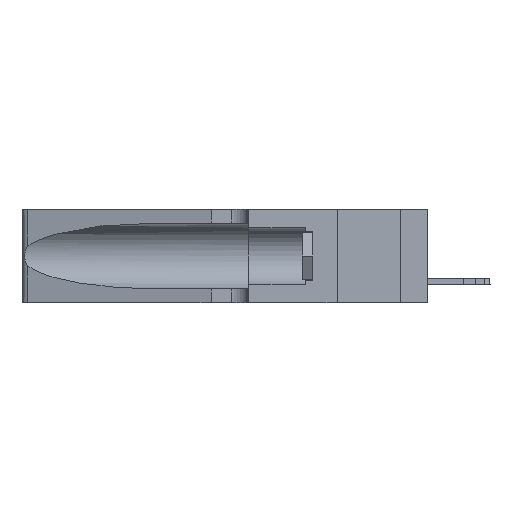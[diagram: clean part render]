
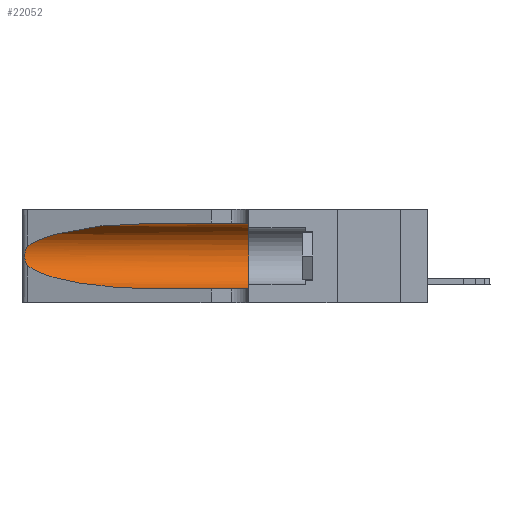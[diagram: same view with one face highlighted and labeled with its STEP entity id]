
A CAD part, left-side view. The second image highlights one B-rep face of the part: STEP entity #22052.
In plain terms, the highlighted cylindrical face has radius 3.308 mm (diameter 6.617 mm), a partial arc.
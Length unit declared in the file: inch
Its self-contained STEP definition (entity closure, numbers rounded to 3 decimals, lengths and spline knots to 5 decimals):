
#426 = CARTESIAN_POINT ( 'NONE',  ( 0.1305, 1.61858, 0.185 ) ) ;
#627 = CARTESIAN_POINT ( 'NONE',  ( 0.1305, 1.61858, 0.05475 ) ) ;
#1019 = EDGE_CURVE ( 'NONE', #13093, #15807, #2407, .T. ) ;
#1480 = CARTESIAN_POINT ( 'NONE',  ( 0.1305, 0.35, 0.31525 ) ) ;
#1628 = CARTESIAN_POINT ( 'NONE',  ( 0.26075, 1.23896, 0.19203 ) ) ;
#2133 = EDGE_CURVE ( 'NONE', #15807, #19721, #5333, .T. ) ;
#2407 =( BOUNDED_CURVE ( )  B_SPLINE_CURVE ( 3, ( #13486, #13326, #16938, #17196 ),
 .UNSPECIFIED., .F., .T. ) 
 B_SPLINE_CURVE_WITH_KNOTS ( ( 4, 4 ),
 ( 3.44316, 4.71239 ),
 .UNSPECIFIED. ) 
 CURVE ( )  GEOMETRIC_REPRESENTATION_ITEM ( )  RATIONAL_B_SPLINE_CURVE ( ( 1., 0.87, 0.87, 1. ) ) 
 REPRESENTATION_ITEM ( '' )  );
#2985 = ORIENTED_EDGE ( 'NONE', *, *, #22074, .T. ) ;
#3859 = CARTESIAN_POINT ( 'NONE',  ( 0.25487, 1.22718, 0.14631 ) ) ;
#4208 = DIRECTION ( 'NONE',  ( 0., -1., 0. ) ) ;
#4405 = EDGE_CURVE ( 'NONE', #7556, #19721, #7891, .T. ) ;
#4512 = DIRECTION ( 'NONE',  ( 0., -1., 0. ) ) ;
#4729 = ORIENTED_EDGE ( 'NONE', *, *, #1019, .T. ) ;
#4730 = VECTOR ( 'NONE', #4208, 39.37008 ) ;
#5333 = LINE ( 'NONE', #627, #22246 ) ;
#5740 = CARTESIAN_POINT ( 'NONE',  ( 0.25639, 1.23186, 0.15144 ) ) ;
#6175 = EDGE_CURVE ( 'NONE', #7309, #13093, #10743, .T. ) ;
#6653 = ORIENTED_EDGE ( 'NONE', *, *, #6175, .T. ) ;
#7309 = VERTEX_POINT ( 'NONE', #8786 ) ;
#7556 = VERTEX_POINT ( 'NONE', #1480 ) ;
#7612 = CARTESIAN_POINT ( 'NONE',  ( 0.1305, 0.35, 0.185 ) ) ;
#7891 = CIRCLE ( 'NONE', #9345, 0.13025 ) ;
#8030 = DIRECTION ( 'NONE',  ( 0., 0., -1. ) ) ;
#8357 = CARTESIAN_POINT ( 'NONE',  ( 0.1305, 0.72297, 0.31525 ) ) ;
#8528 = CARTESIAN_POINT ( 'NONE',  ( 0.2373, 1.15595, 0.28018 ) ) ;
#8786 = CARTESIAN_POINT ( 'NONE',  ( 0.25487, 1.22718, 0.22369 ) ) ;
#9312 = CARTESIAN_POINT ( 'NONE',  ( 0.25555, 1.22993, 0.14849 ) ) ;
#9345 = AXIS2_PLACEMENT_3D ( 'NONE', #7612, #9761, #22788 ) ;
#9389 = CARTESIAN_POINT ( 'NONE',  ( 0.25854, 1.2359, 0.20912 ) ) ;
#9761 = DIRECTION ( 'NONE',  ( 0., 1., 0. ) ) ;
#10060 = LINE ( 'NONE', #13730, #4730 ) ;
#10376 = CARTESIAN_POINT ( 'NONE',  ( 0.25555, 1.22994, 0.2215 ) ) ;
#10743 = B_SPLINE_CURVE_WITH_KNOTS ( 'NONE', 3,
 ( #22916, #10376, #20826, #11388, #9389, #16825, #1628, #13044, #22733, #22653, #24573, #5740, #9312, #3859 ),
 .UNSPECIFIED., .F., .F.,
 ( 4, 2, 2, 2, 2, 2, 4 ),
 ( 0., 0.00027, 0.00053, 0.00107, 0.0016, 0.00187, 0.00214 ),
 .UNSPECIFIED. ) ;
#11388 = CARTESIAN_POINT ( 'NONE',  ( 0.25787, 1.23484, 0.2124 ) ) ;
#11866 = CARTESIAN_POINT ( 'NONE',  ( 0.18966, 0.96281, 0.31525 ) ) ;
#12515 = ORIENTED_EDGE ( 'NONE', *, *, #13778, .F. ) ;
#13044 = CARTESIAN_POINT ( 'NONE',  ( 0.26075, 1.23896, 0.178 ) ) ;
#13093 = VERTEX_POINT ( 'NONE', #14155 ) ;
#13326 = CARTESIAN_POINT ( 'NONE',  ( 0.2373, 1.15595, 0.08982 ) ) ;
#13478 = ORIENTED_EDGE ( 'NONE', *, *, #4405, .F. ) ;
#13486 = CARTESIAN_POINT ( 'NONE',  ( 0.25487, 1.22718, 0.14631 ) ) ;
#13730 = CARTESIAN_POINT ( 'NONE',  ( 0.1305, 1.61858, 0.31525 ) ) ;
#13778 = EDGE_CURVE ( 'NONE', #18638, #7556, #10060, .T. ) ;
#14155 = CARTESIAN_POINT ( 'NONE',  ( 0.25487, 1.22718, 0.14631 ) ) ;
#15198 = ORIENTED_EDGE ( 'NONE', *, *, #2133, .T. ) ;
#15204 = CARTESIAN_POINT ( 'NONE',  ( 0.1305, 0.72297, 0.05475 ) ) ;
#15807 = VERTEX_POINT ( 'NONE', #15204 ) ;
#16825 = CARTESIAN_POINT ( 'NONE',  ( 0.26018, 1.23835, 0.19895 ) ) ;
#16938 = CARTESIAN_POINT ( 'NONE',  ( 0.18966, 0.96281, 0.05475 ) ) ;
#17196 = CARTESIAN_POINT ( 'NONE',  ( 0.1305, 0.72297, 0.05475 ) ) ;
#17886 = AXIS2_PLACEMENT_3D ( 'NONE', #426, #19402, #8030 ) ;
#18638 = VERTEX_POINT ( 'NONE', #8357 ) ;
#19402 = DIRECTION ( 'NONE',  ( 0., -1., 0. ) ) ;
#19721 = VERTEX_POINT ( 'NONE', #21560 ) ;
#20722 = CYLINDRICAL_SURFACE ( 'NONE', #17886, 0.13025 ) ;
#20826 = CARTESIAN_POINT ( 'NONE',  ( 0.25639, 1.23184, 0.21858 ) ) ;
#21012 = FACE_OUTER_BOUND ( 'NONE', #23000, .T. ) ;
#21302 = CARTESIAN_POINT ( 'NONE',  ( 0.1305, 0.72297, 0.31525 ) ) ;
#21560 = CARTESIAN_POINT ( 'NONE',  ( 0.1305, 0.35, 0.05475 ) ) ;
#22052 = ADVANCED_FACE ( 'NONE', ( #21012 ), #20722, .F. ) ;
#22074 = EDGE_CURVE ( 'NONE', #18638, #7309, #22906, .T. ) ;
#22246 = VECTOR ( 'NONE', #4512, 39.37008 ) ;
#22653 = CARTESIAN_POINT ( 'NONE',  ( 0.25856, 1.23593, 0.16098 ) ) ;
#22733 = CARTESIAN_POINT ( 'NONE',  ( 0.26017, 1.23833, 0.17102 ) ) ;
#22788 = DIRECTION ( 'NONE',  ( 0., 0., 1. ) ) ;
#22906 =( BOUNDED_CURVE ( )  B_SPLINE_CURVE ( 3, ( #21302, #11866, #8528, #23616 ),
 .UNSPECIFIED., .F., .F. ) 
 B_SPLINE_CURVE_WITH_KNOTS ( ( 4, 4 ),
 ( 1.5708, 2.84003 ),
 .UNSPECIFIED. ) 
 CURVE ( )  GEOMETRIC_REPRESENTATION_ITEM ( )  RATIONAL_B_SPLINE_CURVE ( ( 1., 0.87, 0.87, 1. ) ) 
 REPRESENTATION_ITEM ( '' )  );
#22916 = CARTESIAN_POINT ( 'NONE',  ( 0.25487, 1.22718, 0.22369 ) ) ;
#23000 = EDGE_LOOP ( 'NONE', ( #2985, #6653, #4729, #15198, #13478, #12515 ) ) ;
#23616 = CARTESIAN_POINT ( 'NONE',  ( 0.25487, 1.22718, 0.22369 ) ) ;
#24573 = CARTESIAN_POINT ( 'NONE',  ( 0.25789, 1.23486, 0.15765 ) ) ;
